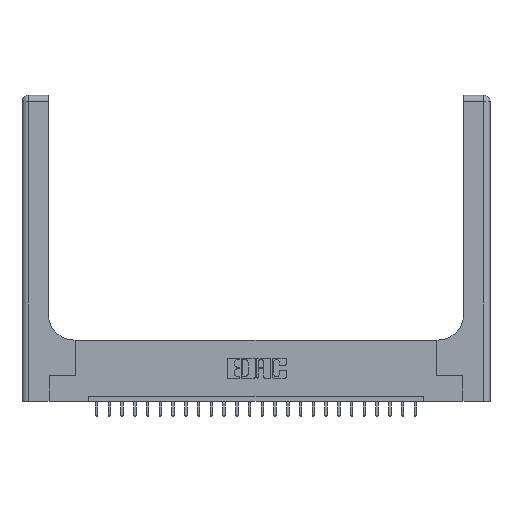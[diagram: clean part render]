
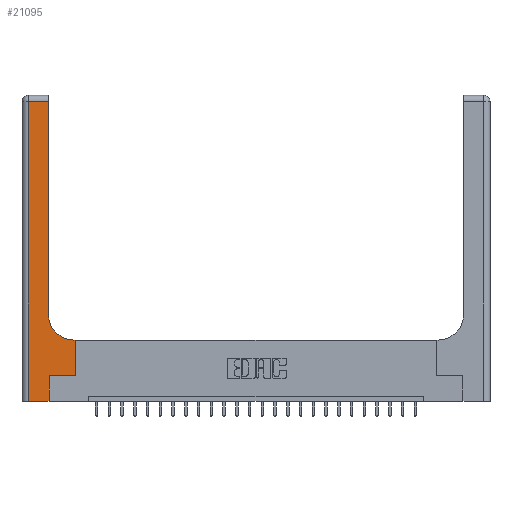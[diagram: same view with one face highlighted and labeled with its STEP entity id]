
A CAD part, top view. The second image highlights one B-rep face of the part: STEP entity #21095.
In plain terms, the highlighted planar face has unit normal (0, 0, 1).
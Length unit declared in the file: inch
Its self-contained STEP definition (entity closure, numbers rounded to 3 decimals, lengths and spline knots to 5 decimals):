
#751 = CARTESIAN_POINT ( 'NONE',  ( 0.265, 0., 0.37 ) ) ;
#958 = CARTESIAN_POINT ( 'NONE',  ( 0.06, 2.94, 0.37 ) ) ;
#1445 = CARTESIAN_POINT ( 'NONE',  ( 0.51, 0.85, 0.37 ) ) ;
#1933 = ORIENTED_EDGE ( 'NONE', *, *, #10320, .T. ) ;
#2707 = CARTESIAN_POINT ( 'NONE',  ( 0.51, 0.6, 0.37 ) ) ;
#3013 = EDGE_CURVE ( 'NONE', #5432, #19226, #12403, .T. ) ;
#3043 = VECTOR ( 'NONE', #11896, 39.37008 ) ;
#3251 = AXIS2_PLACEMENT_3D ( 'NONE', #6530, #10421, #12118 ) ;
#4301 = DIRECTION ( 'NONE',  ( -1., 0., 0. ) ) ;
#4503 = CARTESIAN_POINT ( 'NONE',  ( 0.26, 3., 0.37 ) ) ;
#4761 = ORIENTED_EDGE ( 'NONE', *, *, #10610, .T. ) ;
#4829 = CARTESIAN_POINT ( 'NONE',  ( 0.06, 3., 0.37 ) ) ;
#4881 = VERTEX_POINT ( 'NONE', #958 ) ;
#4937 = ORIENTED_EDGE ( 'NONE', *, *, #19576, .T. ) ;
#5385 = EDGE_CURVE ( 'NONE', #14375, #4881, #9775, .T. ) ;
#5432 = VERTEX_POINT ( 'NONE', #22716 ) ;
#5487 = VECTOR ( 'NONE', #7056, 39.37008 ) ;
#5598 = AXIS2_PLACEMENT_3D ( 'NONE', #1445, #18265, #14501 ) ;
#6421 = VERTEX_POINT ( 'NONE', #21422 ) ;
#6438 = DIRECTION ( 'NONE',  ( 0., 1., 0. ) ) ;
#6530 = CARTESIAN_POINT ( 'NONE',  ( 0., 3., 0.37 ) ) ;
#7056 = DIRECTION ( 'NONE',  ( -1., 0., 0. ) ) ;
#7204 = LINE ( 'NONE', #21979, #17876 ) ;
#8606 = EDGE_CURVE ( 'NONE', #11225, #14375, #16978, .T. ) ;
#8668 = EDGE_CURVE ( 'NONE', #6421, #19549, #21080, .T. ) ;
#8825 = ORIENTED_EDGE ( 'NONE', *, *, #5385, .T. ) ;
#9693 = FACE_OUTER_BOUND ( 'NONE', #20466, .T. ) ;
#9775 = LINE ( 'NONE', #13504, #22709 ) ;
#9960 = DIRECTION ( 'NONE',  ( 0., 1., 0. ) ) ;
#10293 = DIRECTION ( 'NONE',  ( 0., -1., 0. ) ) ;
#10320 = EDGE_CURVE ( 'NONE', #19549, #13151, #10324, .T. ) ;
#10324 = LINE ( 'NONE', #12369, #15245 ) ;
#10421 = DIRECTION ( 'NONE',  ( 0., 0., -1. ) ) ;
#10488 = EDGE_CURVE ( 'NONE', #4881, #6421, #20919, .T. ) ;
#10610 = EDGE_CURVE ( 'NONE', #19226, #11225, #23776, .T. ) ;
#10771 = VECTOR ( 'NONE', #6438, 39.37008 ) ;
#10954 = VECTOR ( 'NONE', #16240, 39.37008 ) ;
#11225 = VERTEX_POINT ( 'NONE', #18819 ) ;
#11896 = DIRECTION ( 'NONE',  ( 1., 0., 0. ) ) ;
#12118 = DIRECTION ( 'NONE',  ( -1., 0., 0. ) ) ;
#12145 = LINE ( 'NONE', #16120, #10954 ) ;
#12369 = CARTESIAN_POINT ( 'NONE',  ( 0.265, 0., 0.37 ) ) ;
#12403 = LINE ( 'NONE', #19785, #5487 ) ;
#13146 = ORIENTED_EDGE ( 'NONE', *, *, #3013, .T. ) ;
#13151 = VERTEX_POINT ( 'NONE', #22918 ) ;
#13504 = CARTESIAN_POINT ( 'NONE',  ( 0., 2.94, 0.37 ) ) ;
#13938 = CARTESIAN_POINT ( 'NONE',  ( 0.528, 0.25, 0.37 ) ) ;
#14375 = VERTEX_POINT ( 'NONE', #18579 ) ;
#14501 = DIRECTION ( 'NONE',  ( 1., 0., 0. ) ) ;
#14880 = ORIENTED_EDGE ( 'NONE', *, *, #8606, .T. ) ;
#15245 = VECTOR ( 'NONE', #9960, 39.37008 ) ;
#16007 = VERTEX_POINT ( 'NONE', #13938 ) ;
#16120 = CARTESIAN_POINT ( 'NONE',  ( 0.265, 0.25, 0.37 ) ) ;
#16240 = DIRECTION ( 'NONE',  ( 1., 0., 0. ) ) ;
#16978 = LINE ( 'NONE', #4503, #10771 ) ;
#17203 = VECTOR ( 'NONE', #10293, 39.37008 ) ;
#17390 = ORIENTED_EDGE ( 'NONE', *, *, #8668, .T. ) ;
#17876 = VECTOR ( 'NONE', #23671, 39.37008 ) ;
#18265 = DIRECTION ( 'NONE',  ( 0., 0., -1. ) ) ;
#18579 = CARTESIAN_POINT ( 'NONE',  ( 0.26, 2.94, 0.37 ) ) ;
#18798 = CARTESIAN_POINT ( 'NONE',  ( 0., 0., 0.37 ) ) ;
#18819 = CARTESIAN_POINT ( 'NONE',  ( 0.26, 0.85, 0.37 ) ) ;
#18968 = EDGE_CURVE ( 'NONE', #16007, #5432, #7204, .T. ) ;
#19226 = VERTEX_POINT ( 'NONE', #2707 ) ;
#19549 = VERTEX_POINT ( 'NONE', #751 ) ;
#19576 = EDGE_CURVE ( 'NONE', #13151, #16007, #12145, .T. ) ;
#19785 = CARTESIAN_POINT ( 'NONE',  ( 0.26, 0.6, 0.37 ) ) ;
#20466 = EDGE_LOOP ( 'NONE', ( #14880, #8825, #20754, #17390, #1933, #4937, #21763, #13146, #4761 ) ) ;
#20754 = ORIENTED_EDGE ( 'NONE', *, *, #10488, .T. ) ;
#20808 = PLANE ( 'NONE',  #3251 ) ;
#20919 = LINE ( 'NONE', #4829, #17203 ) ;
#21080 = LINE ( 'NONE', #18798, #3043 ) ;
#21095 = ADVANCED_FACE ( 'NONE', ( #9693 ), #20808, .F. ) ;
#21422 = CARTESIAN_POINT ( 'NONE',  ( 0.06, 0., 0.37 ) ) ;
#21763 = ORIENTED_EDGE ( 'NONE', *, *, #18968, .T. ) ;
#21979 = CARTESIAN_POINT ( 'NONE',  ( 0.528, 0.25, 0.37 ) ) ;
#22709 = VECTOR ( 'NONE', #4301, 39.37008 ) ;
#22716 = CARTESIAN_POINT ( 'NONE',  ( 0.528, 0.6, 0.37 ) ) ;
#22918 = CARTESIAN_POINT ( 'NONE',  ( 0.265, 0.25, 0.37 ) ) ;
#23671 = DIRECTION ( 'NONE',  ( 0., 1., 0. ) ) ;
#23776 = CIRCLE ( 'NONE', #5598, 0.25 ) ;
